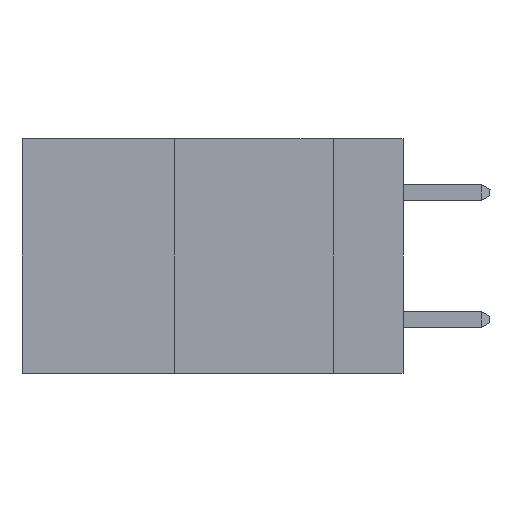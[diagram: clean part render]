
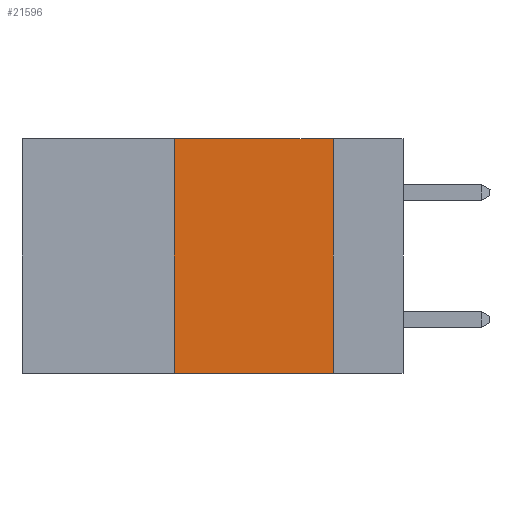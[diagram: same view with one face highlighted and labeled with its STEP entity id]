
A CAD part, left-side view. The second image highlights one B-rep face of the part: STEP entity #21596.
In plain terms, the highlighted planar face has unit normal (-1, 0, 0).
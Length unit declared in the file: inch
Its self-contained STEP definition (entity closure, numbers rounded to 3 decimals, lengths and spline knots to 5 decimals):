
#52 = CARTESIAN_POINT ( 'NONE',  ( 0., 0.11, -0.37 ) ) ;
#347 = CARTESIAN_POINT ( 'NONE',  ( 0., 0.11, 0. ) ) ;
#354 = ORIENTED_EDGE ( 'NONE', *, *, #12684, .F. ) ;
#1244 = LINE ( 'NONE', #3577, #7985 ) ;
#2824 = FACE_OUTER_BOUND ( 'NONE', #17926, .T. ) ;
#2890 = ORIENTED_EDGE ( 'NONE', *, *, #16513, .F. ) ;
#3396 = DIRECTION ( 'NONE',  ( 0., -1., 0. ) ) ;
#3569 = CARTESIAN_POINT ( 'NONE',  ( 0., 0.6, 0. ) ) ;
#3577 = CARTESIAN_POINT ( 'NONE',  ( 0., 0.11, 0. ) ) ;
#3977 = DIRECTION ( 'NONE',  ( 0., 0., 1. ) ) ;
#4006 = VERTEX_POINT ( 'NONE', #52 ) ;
#4532 = VERTEX_POINT ( 'NONE', #20953 ) ;
#5125 = VERTEX_POINT ( 'NONE', #347 ) ;
#5534 = VECTOR ( 'NONE', #3977, 39.37008 ) ;
#5551 = EDGE_CURVE ( 'NONE', #5125, #4006, #1244, .T. ) ;
#6838 = CARTESIAN_POINT ( 'NONE',  ( 0., 0.6, -0.37 ) ) ;
#7667 = VECTOR ( 'NONE', #3396, 39.37008 ) ;
#7985 = VECTOR ( 'NONE', #9240, 39.37008 ) ;
#9240 = DIRECTION ( 'NONE',  ( 0., 0., -1. ) ) ;
#9492 = DIRECTION ( 'NONE',  ( 0., -1., 0. ) ) ;
#10887 = ORIENTED_EDGE ( 'NONE', *, *, #24299, .T. ) ;
#11043 = VERTEX_POINT ( 'NONE', #11400 ) ;
#11400 = CARTESIAN_POINT ( 'NONE',  ( 0., 0.36, -0.37 ) ) ;
#11511 = DIRECTION ( 'NONE',  ( 1., 0., 0. ) ) ;
#11619 = LINE ( 'NONE', #6838, #7667 ) ;
#12684 = EDGE_CURVE ( 'NONE', #4532, #5125, #14541, .T. ) ;
#13290 = CARTESIAN_POINT ( 'NONE',  ( 0., 0.6, 0. ) ) ;
#13470 = PLANE ( 'NONE',  #18075 ) ;
#13623 = DIRECTION ( 'NONE',  ( 0., 0., -1. ) ) ;
#14541 = LINE ( 'NONE', #13290, #19089 ) ;
#15899 = LINE ( 'NONE', #17766, #5534 ) ;
#16513 = EDGE_CURVE ( 'NONE', #11043, #4532, #15899, .T. ) ;
#17766 = CARTESIAN_POINT ( 'NONE',  ( 0., 0.36, 0. ) ) ;
#17926 = EDGE_LOOP ( 'NONE', ( #21243, #354, #2890, #10887 ) ) ;
#18075 = AXIS2_PLACEMENT_3D ( 'NONE', #3569, #11511, #13623 ) ;
#19089 = VECTOR ( 'NONE', #9492, 39.37008 ) ;
#20953 = CARTESIAN_POINT ( 'NONE',  ( 0., 0.36, 0. ) ) ;
#21243 = ORIENTED_EDGE ( 'NONE', *, *, #5551, .F. ) ;
#21596 = ADVANCED_FACE ( 'NONE', ( #2824 ), #13470, .F. ) ;
#24299 = EDGE_CURVE ( 'NONE', #11043, #4006, #11619, .T. ) ;
